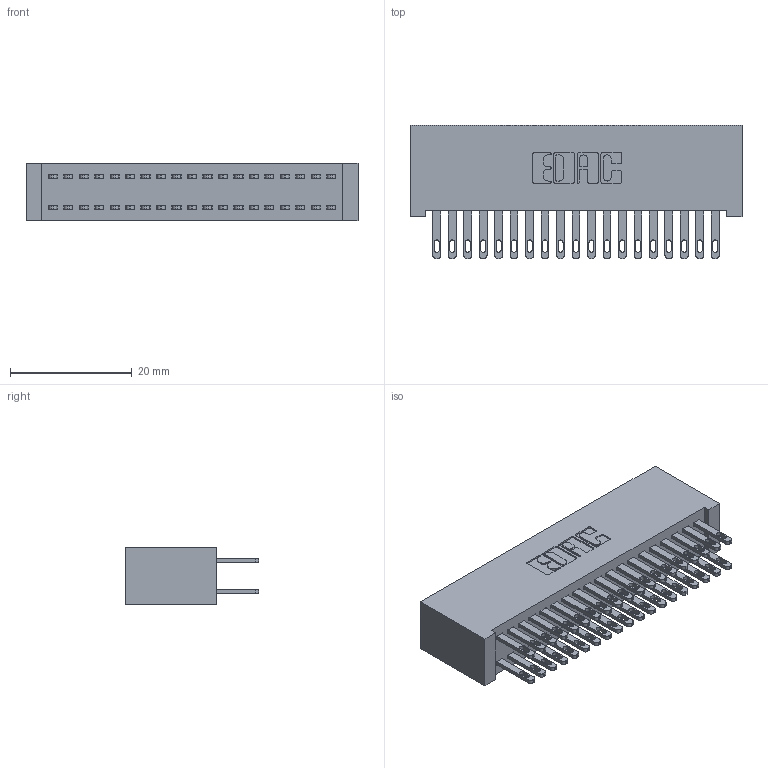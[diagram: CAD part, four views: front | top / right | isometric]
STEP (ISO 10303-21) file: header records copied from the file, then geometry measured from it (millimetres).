
FILE_DESCRIPTION (( 'STEP AP203' ), '1' );
FILE_NAME ('342-038-500-201.STEP', '2018-08-11T21:40:23', ( '' ), ( '' ), 'SwSTEP 2.0', 'SolidWorks 2016', '' );
FILE_SCHEMA (( 'CONFIG_CONTROL_DESIGN' ));
Length unit declared in the file: inch
Products named in the file (3): 342-038-500-201; 342 Part_Lugless; 345-292-001_345-293-100
Assembly tree (39 placements, depth 2):
  342-038-500-201
    342 Part_Lugless
    345-292-001_345-293-100  x38
Bounding box: 54.51 x 21.85 x 9.4 mm (x, y, z)
Volume: 5344.3 mm3; surface area: 8942.6 mm2
Topology: 39 solids, 39 shells, 1926 faces, 5861 edges, 3906 vertices
Faces by surface type: plane 1202, cylinder 724
Entity records: 14719 total; most frequent: CARTESIAN_POINT 2462, ORIENTED_EDGE 2398, DIRECTION 2139, EDGE_CURVE 1199, VECTOR 1075, LINE 1075, VERTEX_POINT 798, AXIS2_PLACEMENT_3D 532
